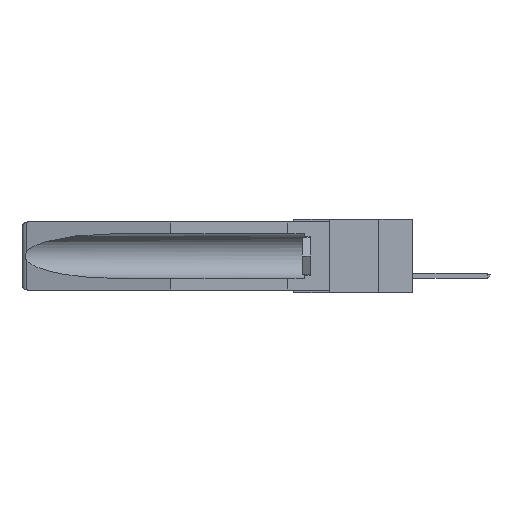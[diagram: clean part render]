
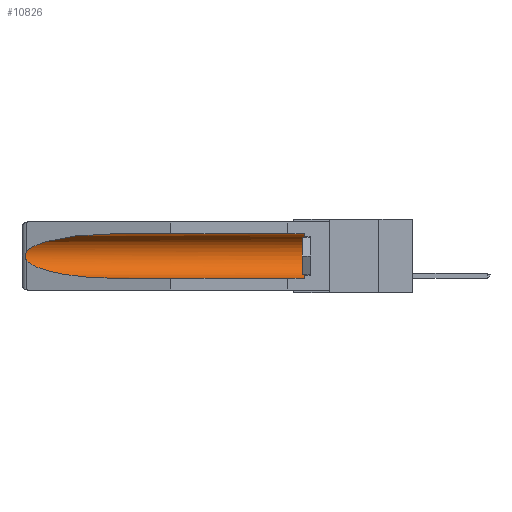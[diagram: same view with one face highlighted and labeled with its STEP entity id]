
A CAD part, left-side view. The second image highlights one B-rep face of the part: STEP entity #10826.
In plain terms, the highlighted cylindrical face has radius 2.857 mm (diameter 5.715 mm), a partial arc.
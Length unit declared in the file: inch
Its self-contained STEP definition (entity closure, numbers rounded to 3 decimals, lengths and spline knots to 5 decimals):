
#143 = EDGE_CURVE ( 'NONE', #12405, #7351, #19142, .T. ) ;
#241 = CARTESIAN_POINT ( 'NONE',  ( 0.155, 1.07973, -0.284 ) ) ;
#444 = EDGE_CURVE ( 'NONE', #4684, #10251, #19548, .T. ) ;
#464 = CARTESIAN_POINT ( 'NONE',  ( 0.26597, 1.5296, -0.19026 ) ) ;
#487 = CARTESIAN_POINT ( 'NONE',  ( 0.21114, 1.30732, -0.059 ) ) ;
#666 = CARTESIAN_POINT ( 'NONE',  ( 0.26537, 1.52718, -0.14972 ) ) ;
#758 = CARTESIAN_POINT ( 'NONE',  ( 0.155, -0.30754, -0.284 ) ) ;
#1034 = AXIS2_PLACEMENT_3D ( 'NONE', #17896, #8224, #9942 ) ;
#1575 = EDGE_LOOP ( 'NONE', ( #13852, #9423, #18601, #20715, #12052, #3036 ) ) ;
#1727 = EDGE_CURVE ( 'NONE', #11509, #12405, #6989, .T. ) ;
#1766 = CYLINDRICAL_SURFACE ( 'NONE', #16553, 0.1125 ) ;
#2486 = EDGE_CURVE ( 'NONE', #10251, #10493, #8868, .T. ) ;
#2682 = VECTOR ( 'NONE', #8660, 39.37008 ) ;
#3036 = ORIENTED_EDGE ( 'NONE', *, *, #2486, .T. ) ;
#3212 = CARTESIAN_POINT ( 'NONE',  ( 0.25451, 1.48313, -0.24835 ) ) ;
#3443 = CARTESIAN_POINT ( 'NONE',  ( 0.26537, 1.52718, -0.14972 ) ) ;
#3605 = CARTESIAN_POINT ( 'NONE',  ( 0.155, 1.07973, -0.059 ) ) ;
#3740 = CARTESIAN_POINT ( 'NONE',  ( 0.155, -0.30754, -0.1715 ) ) ;
#4684 = VERTEX_POINT ( 'NONE', #5478 ) ;
#4820 = CARTESIAN_POINT ( 'NONE',  ( 0.155, 0.126, -0.059 ) ) ;
#5059 = CARTESIAN_POINT ( 'NONE',  ( 0.2673, 1.5327, -0.16383 ) ) ;
#5478 = CARTESIAN_POINT ( 'NONE',  ( 0.155, 0.126, -0.284 ) ) ;
#6206 = CARTESIAN_POINT ( 'NONE',  ( 0.26537, 1.52718, -0.19328 ) ) ;
#6854 = VECTOR ( 'NONE', #13630, 39.37008 ) ;
#6947 = CARTESIAN_POINT ( 'NONE',  ( 0.2675, 1.53308, -0.17534 ) ) ;
#6989 = B_SPLINE_CURVE_WITH_KNOTS ( 'NONE', 3,
 ( #3443, #19724, #8429, #5059, #10088, #6947, #13393, #13251, #464, #10158 ),
 .UNSPECIFIED., .F., .F.,
 ( 4, 2, 2, 2, 4 ),
 ( 0., 0.00029, 0.00058, 0.00087, 0.00117 ),
 .UNSPECIFIED. ) ;
#7351 = VERTEX_POINT ( 'NONE', #16262 ) ;
#7779 = LINE ( 'NONE', #758, #2682 ) ;
#8224 = DIRECTION ( 'NONE',  ( 0., -1., 0. ) ) ;
#8429 = CARTESIAN_POINT ( 'NONE',  ( 0.26654, 1.53092, -0.15636 ) ) ;
#8490 = CARTESIAN_POINT ( 'NONE',  ( 0.21114, 1.30732, -0.284 ) ) ;
#8660 = DIRECTION ( 'NONE',  ( 0., 1., 0. ) ) ;
#8803 = CARTESIAN_POINT ( 'NONE',  ( 0.25451, 1.48313, -0.09465 ) ) ;
#8868 = LINE ( 'NONE', #18687, #6854 ) ;
#9197 =( BOUNDED_CURVE ( )  B_SPLINE_CURVE ( 3, ( #3605, #487, #8803, #12215 ),
 .UNSPECIFIED., .F., .F. ) 
 B_SPLINE_CURVE_WITH_KNOTS ( ( 4, 4 ),
 ( 4.71239, 6.08839 ),
 .UNSPECIFIED. ) 
 CURVE ( )  GEOMETRIC_REPRESENTATION_ITEM ( )  RATIONAL_B_SPLINE_CURVE ( ( 1., 0.848, 0.848, 1. ) ) 
 REPRESENTATION_ITEM ( '' )  );
#9423 = ORIENTED_EDGE ( 'NONE', *, *, #1727, .T. ) ;
#9942 = DIRECTION ( 'NONE',  ( 0., 0., 1. ) ) ;
#10088 = CARTESIAN_POINT ( 'NONE',  ( 0.2675, 1.53308, -0.16763 ) ) ;
#10158 = CARTESIAN_POINT ( 'NONE',  ( 0.26537, 1.52718, -0.19328 ) ) ;
#10181 = DIRECTION ( 'NONE',  ( 0., 1., 0. ) ) ;
#10184 = CARTESIAN_POINT ( 'NONE',  ( 0.26537, 1.52718, -0.19328 ) ) ;
#10186 = FACE_OUTER_BOUND ( 'NONE', #1575, .T. ) ;
#10251 = VERTEX_POINT ( 'NONE', #4820 ) ;
#10493 = VERTEX_POINT ( 'NONE', #11236 ) ;
#10826 = ADVANCED_FACE ( 'NONE', ( #10186 ), #1766, .F. ) ;
#10919 = EDGE_CURVE ( 'NONE', #10493, #11509, #9197, .T. ) ;
#11236 = CARTESIAN_POINT ( 'NONE',  ( 0.155, 1.07973, -0.059 ) ) ;
#11509 = VERTEX_POINT ( 'NONE', #666 ) ;
#12052 = ORIENTED_EDGE ( 'NONE', *, *, #444, .T. ) ;
#12215 = CARTESIAN_POINT ( 'NONE',  ( 0.26537, 1.52718, -0.14972 ) ) ;
#12405 = VERTEX_POINT ( 'NONE', #10184 ) ;
#13251 = CARTESIAN_POINT ( 'NONE',  ( 0.26655, 1.53094, -0.18657 ) ) ;
#13393 = CARTESIAN_POINT ( 'NONE',  ( 0.2673, 1.53269, -0.17917 ) ) ;
#13479 = EDGE_CURVE ( 'NONE', #4684, #7351, #7779, .T. ) ;
#13630 = DIRECTION ( 'NONE',  ( 0., 1., 0. ) ) ;
#13852 = ORIENTED_EDGE ( 'NONE', *, *, #10919, .T. ) ;
#15111 = DIRECTION ( 'NONE',  ( 0., 0., 1. ) ) ;
#16262 = CARTESIAN_POINT ( 'NONE',  ( 0.155, 1.07973, -0.284 ) ) ;
#16553 = AXIS2_PLACEMENT_3D ( 'NONE', #3740, #10181, #15111 ) ;
#17896 = CARTESIAN_POINT ( 'NONE',  ( 0.155, 0.126, -0.1715 ) ) ;
#18601 = ORIENTED_EDGE ( 'NONE', *, *, #143, .T. ) ;
#18687 = CARTESIAN_POINT ( 'NONE',  ( 0.155, -0.30754, -0.059 ) ) ;
#19142 =( BOUNDED_CURVE ( )  B_SPLINE_CURVE ( 3, ( #6206, #3212, #8490, #241 ),
 .UNSPECIFIED., .F., .F. ) 
 B_SPLINE_CURVE_WITH_KNOTS ( ( 4, 4 ),
 ( 0.1948, 1.5708 ),
 .UNSPECIFIED. ) 
 CURVE ( )  GEOMETRIC_REPRESENTATION_ITEM ( )  RATIONAL_B_SPLINE_CURVE ( ( 1., 0.848, 0.848, 1. ) ) 
 REPRESENTATION_ITEM ( '' )  );
#19548 = CIRCLE ( 'NONE', #1034, 0.1125 ) ;
#19724 = CARTESIAN_POINT ( 'NONE',  ( 0.26597, 1.52961, -0.15275 ) ) ;
#20715 = ORIENTED_EDGE ( 'NONE', *, *, #13479, .F. ) ;
